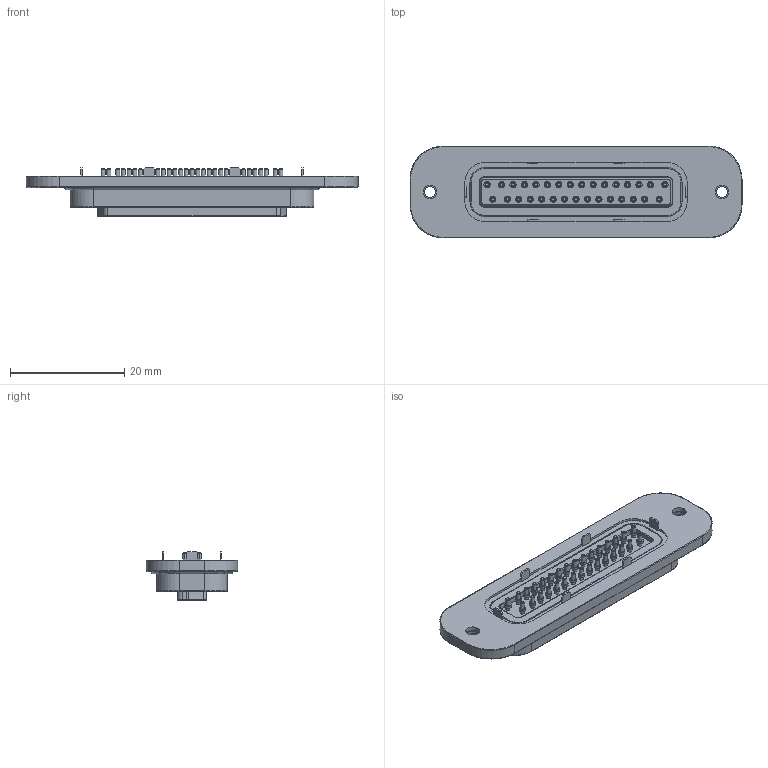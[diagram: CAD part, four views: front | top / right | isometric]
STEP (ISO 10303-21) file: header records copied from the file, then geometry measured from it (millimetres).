
FILE_DESCRIPTION (( 'STEP AP214' ), '1' );
FILE_NAME ('686A3131260114E.STEP', '2023-04-26T16:20:49', ( '' ), ( '' ), 'SwSTEP 2.0', 'SolidWorks 2020', '' );
FILE_SCHEMA (( 'AUTOMOTIVE_DESIGN' ));
Length unit declared in the file: millimetre
Products named in the file (1): 686A3131260114E
Bounding box: 58 x 16.04 x 8.55 mm (x, y, z)
Volume: 3604 mm3; surface area: 4555.2 mm2
Topology: 2 solids, 2 shells, 913 faces, 2066 edges, 1260 vertices
Faces by surface type: cylinder 433, plane 263, cone 167, bspline 50
Entity records: 35996 total; most frequent: CARTESIAN_POINT 5234, DIRECTION 4735, ORIENTED_EDGE 3946, EDGE_CURVE 1973, AXIS2_PLACEMENT_3D 1941, VERTEX_POINT 1260, EDGE_LOOP 1115, CIRCLE 1077
